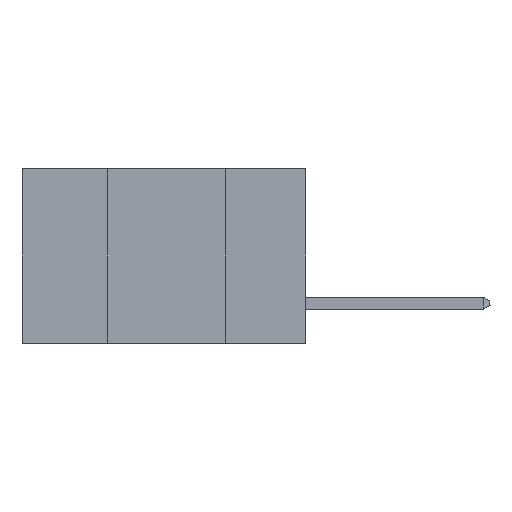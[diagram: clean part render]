
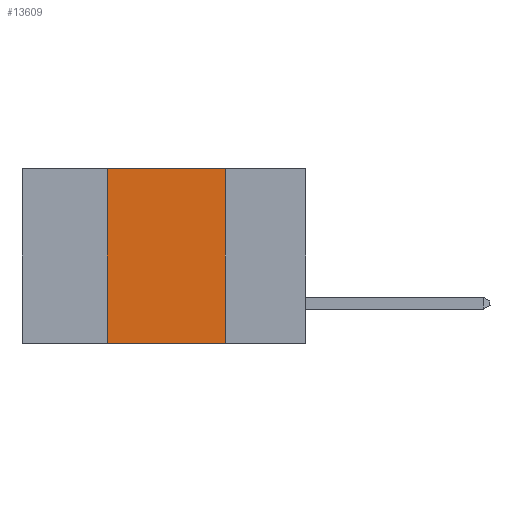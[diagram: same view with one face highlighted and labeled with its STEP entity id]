
A CAD part, left-side view. The second image highlights one B-rep face of the part: STEP entity #13609.
In plain terms, the highlighted planar face has unit normal (-1, 0, 0).
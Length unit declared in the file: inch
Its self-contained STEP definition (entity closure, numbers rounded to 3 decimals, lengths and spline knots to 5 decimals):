
#440 = EDGE_LOOP ( 'NONE', ( #11615, #10144, #925, #3881 ) ) ;
#603 = DIRECTION ( 'NONE',  ( 0., 0., -1. ) ) ;
#632 = VECTOR ( 'NONE', #13988, 39.37008 ) ;
#925 = ORIENTED_EDGE ( 'NONE', *, *, #5254, .F. ) ;
#2873 = DIRECTION ( 'NONE',  ( 0., -1., 0. ) ) ;
#3264 = EDGE_CURVE ( 'NONE', #4547, #7521, #13755, .T. ) ;
#3369 = VECTOR ( 'NONE', #10004, 39.37008 ) ;
#3385 = DIRECTION ( 'NONE',  ( 0., 0., -1. ) ) ;
#3458 = VERTEX_POINT ( 'NONE', #13862 ) ;
#3881 = ORIENTED_EDGE ( 'NONE', *, *, #3264, .T. ) ;
#3927 = CARTESIAN_POINT ( 'NONE',  ( 0., 0.6, 0. ) ) ;
#4119 = DIRECTION ( 'NONE',  ( 1., 0., 0. ) ) ;
#4260 = VERTEX_POINT ( 'NONE', #13087 ) ;
#4351 = EDGE_CURVE ( 'NONE', #3458, #7521, #7475, .T. ) ;
#4547 = VERTEX_POINT ( 'NONE', #14542 ) ;
#5065 = CARTESIAN_POINT ( 'NONE',  ( 0., 0.42, 0. ) ) ;
#5254 = EDGE_CURVE ( 'NONE', #4547, #4260, #9946, .T. ) ;
#6045 = VECTOR ( 'NONE', #2873, 39.37008 ) ;
#6765 = LINE ( 'NONE', #8106, #6045 ) ;
#7163 = CARTESIAN_POINT ( 'NONE',  ( 0., 0.17, -0.37 ) ) ;
#7475 = LINE ( 'NONE', #8085, #11218 ) ;
#7521 = VERTEX_POINT ( 'NONE', #7163 ) ;
#7700 = CARTESIAN_POINT ( 'NONE',  ( 0., 0.6, -0.37 ) ) ;
#8085 = CARTESIAN_POINT ( 'NONE',  ( 0., 0.17, 0. ) ) ;
#8106 = CARTESIAN_POINT ( 'NONE',  ( 0., 0.6, 0. ) ) ;
#8303 = FACE_OUTER_BOUND ( 'NONE', #440, .T. ) ;
#9636 = PLANE ( 'NONE',  #9886 ) ;
#9886 = AXIS2_PLACEMENT_3D ( 'NONE', #3927, #4119, #603 ) ;
#9946 = LINE ( 'NONE', #5065, #632 ) ;
#10004 = DIRECTION ( 'NONE',  ( 0., -1., 0. ) ) ;
#10144 = ORIENTED_EDGE ( 'NONE', *, *, #10937, .F. ) ;
#10937 = EDGE_CURVE ( 'NONE', #4260, #3458, #6765, .T. ) ;
#11218 = VECTOR ( 'NONE', #3385, 39.37008 ) ;
#11615 = ORIENTED_EDGE ( 'NONE', *, *, #4351, .F. ) ;
#13087 = CARTESIAN_POINT ( 'NONE',  ( 0., 0.42, 0. ) ) ;
#13609 = ADVANCED_FACE ( 'NONE', ( #8303 ), #9636, .F. ) ;
#13755 = LINE ( 'NONE', #7700, #3369 ) ;
#13862 = CARTESIAN_POINT ( 'NONE',  ( 0., 0.17, 0. ) ) ;
#13988 = DIRECTION ( 'NONE',  ( 0., 0., 1. ) ) ;
#14542 = CARTESIAN_POINT ( 'NONE',  ( 0., 0.42, -0.37 ) ) ;
